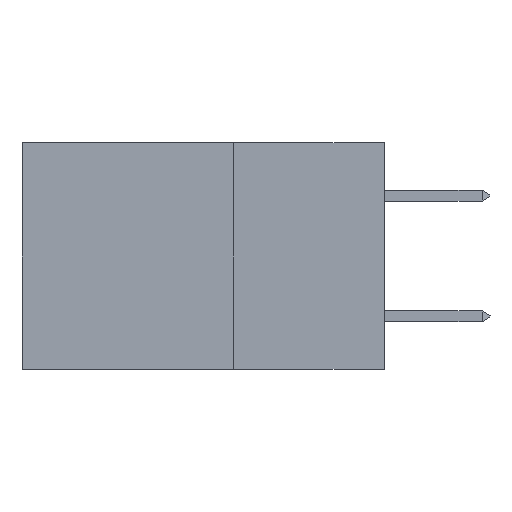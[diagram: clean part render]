
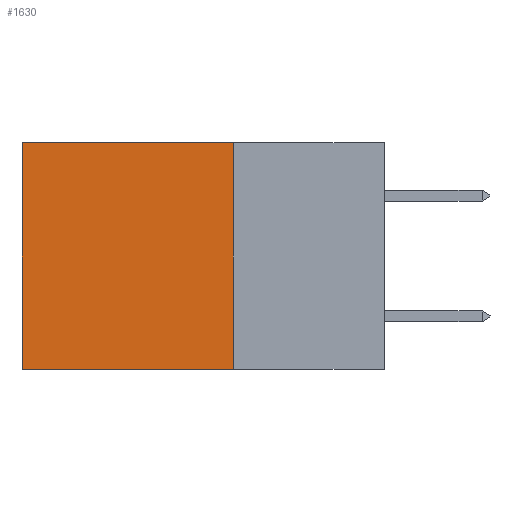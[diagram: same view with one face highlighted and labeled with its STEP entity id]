
A CAD part, left-side view. The second image highlights one B-rep face of the part: STEP entity #1630.
In plain terms, the highlighted planar face has unit normal (-1, 0, 0).
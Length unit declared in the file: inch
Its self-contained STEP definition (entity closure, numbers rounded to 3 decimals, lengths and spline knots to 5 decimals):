
#278 = PLANE ( 'NONE',  #7426 ) ;
#292 = CARTESIAN_POINT ( 'NONE',  ( 0.2875, 0.25, 0. ) ) ;
#640 = CARTESIAN_POINT ( 'NONE',  ( 0.2875, 0.25, -0.375 ) ) ;
#1157 = LINE ( 'NONE', #8476, #7991 ) ;
#1187 = EDGE_CURVE ( 'NONE', #6126, #2437, #16672, .T. ) ;
#1630 = ADVANCED_FACE ( 'NONE', ( #14005 ), #278, .F. ) ;
#2167 = EDGE_LOOP ( 'NONE', ( #19319, #9419, #14271, #19557 ) ) ;
#2437 = VERTEX_POINT ( 'NONE', #2646 ) ;
#2646 = CARTESIAN_POINT ( 'NONE',  ( 0.2875, 0.6, -0.375 ) ) ;
#3889 = EDGE_CURVE ( 'NONE', #19841, #14868, #12811, .T. ) ;
#4921 = CARTESIAN_POINT ( 'NONE',  ( 0.2875, 0.25, -0.375 ) ) ;
#5125 = DIRECTION ( 'NONE',  ( 1., 0., 0. ) ) ;
#5793 = DIRECTION ( 'NONE',  ( 0., 1., 0. ) ) ;
#6126 = VERTEX_POINT ( 'NONE', #8011 ) ;
#7426 = AXIS2_PLACEMENT_3D ( 'NONE', #4921, #5125, #9543 ) ;
#7479 = VECTOR ( 'NONE', #14596, 39.37008 ) ;
#7991 = VECTOR ( 'NONE', #13217, 39.37008 ) ;
#8011 = CARTESIAN_POINT ( 'NONE',  ( 0.2875, 0.25, -0.375 ) ) ;
#8476 = CARTESIAN_POINT ( 'NONE',  ( 0.2875, 0.6, -0.375 ) ) ;
#9419 = ORIENTED_EDGE ( 'NONE', *, *, #1187, .F. ) ;
#9543 = DIRECTION ( 'NONE',  ( 0., 0., -1. ) ) ;
#10366 = CARTESIAN_POINT ( 'NONE',  ( 0.2875, 0.6, 0. ) ) ;
#10633 = LINE ( 'NONE', #640, #7479 ) ;
#11173 = EDGE_CURVE ( 'NONE', #14868, #2437, #1157, .T. ) ;
#11837 = VECTOR ( 'NONE', #19640, 39.37008 ) ;
#12811 = LINE ( 'NONE', #13810, #17136 ) ;
#13217 = DIRECTION ( 'NONE',  ( 0., 0., -1. ) ) ;
#13810 = CARTESIAN_POINT ( 'NONE',  ( 0.2875, 0.25, 0. ) ) ;
#14005 = FACE_OUTER_BOUND ( 'NONE', #2167, .T. ) ;
#14271 = ORIENTED_EDGE ( 'NONE', *, *, #18619, .F. ) ;
#14596 = DIRECTION ( 'NONE',  ( 0., 0., -1. ) ) ;
#14868 = VERTEX_POINT ( 'NONE', #10366 ) ;
#16275 = CARTESIAN_POINT ( 'NONE',  ( 0.2875, 0.25, -0.375 ) ) ;
#16672 = LINE ( 'NONE', #16275, #11837 ) ;
#17136 = VECTOR ( 'NONE', #5793, 39.37008 ) ;
#18619 = EDGE_CURVE ( 'NONE', #19841, #6126, #10633, .T. ) ;
#19319 = ORIENTED_EDGE ( 'NONE', *, *, #11173, .T. ) ;
#19557 = ORIENTED_EDGE ( 'NONE', *, *, #3889, .T. ) ;
#19640 = DIRECTION ( 'NONE',  ( 0., 1., 0. ) ) ;
#19841 = VERTEX_POINT ( 'NONE', #292 ) ;
